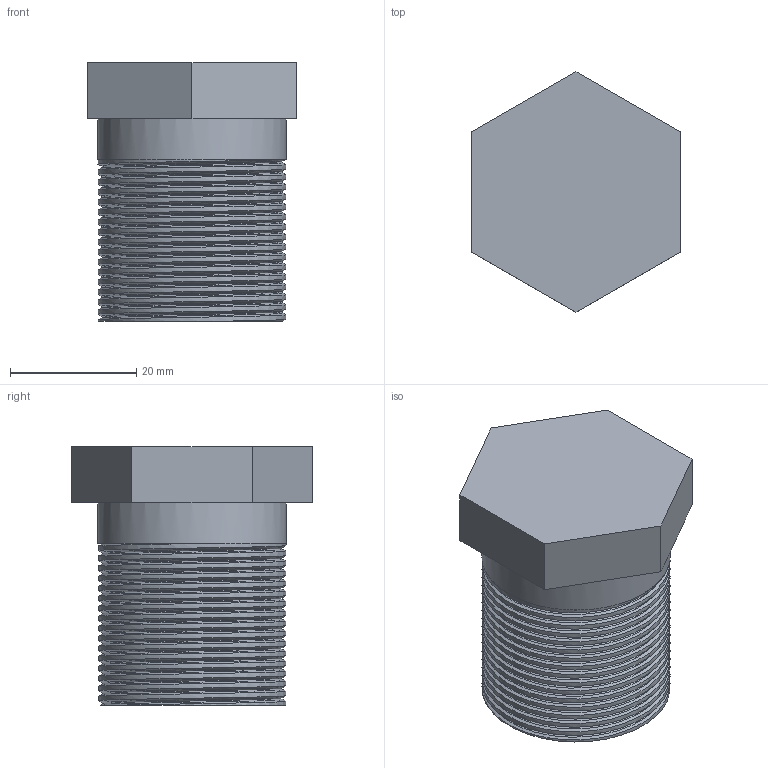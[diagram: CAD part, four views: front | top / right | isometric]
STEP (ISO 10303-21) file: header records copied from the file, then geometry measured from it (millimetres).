
FILE_DESCRIPTION(('FreeCAD Model'),'2;1');
FILE_NAME('buffer bolt sized.step','2016-02-26T23:06:04',('Author'),(''), 'Open CASCADE STEP processor 6.8','FreeCAD','Unknown');
FILE_SCHEMA(('AUTOMOTIVE_DESIGN_CC2 { 1 2 10303 214 -1 1 5 4 }'));
Products named in the file (1): Pocket
Bounding box: 33 x 38.1 x 40.94 mm (x, y, z)
Volume: 23308.2 mm3; surface area: 8754.2 mm2
Topology: 1 solids, 1 shells, 120 faces, 345 edges, 230 vertices
Faces by surface type: plane 46, cylinder 37, bspline 37
Full cylindrical faces by diameter (mm): 17.33 x1, 17.677 x1, 29.845 x1
Entity records: 56911 total; most frequent: CARTESIAN_POINT 51700, B_SPLINE_CURVE_WITH_KNOTS 816, ORIENTED_EDGE 690, PCURVE 690, DEFINITIONAL_REPRESENTATION 690, DIRECTION 388, EDGE_CURVE 345, SURFACE_CURVE 342
